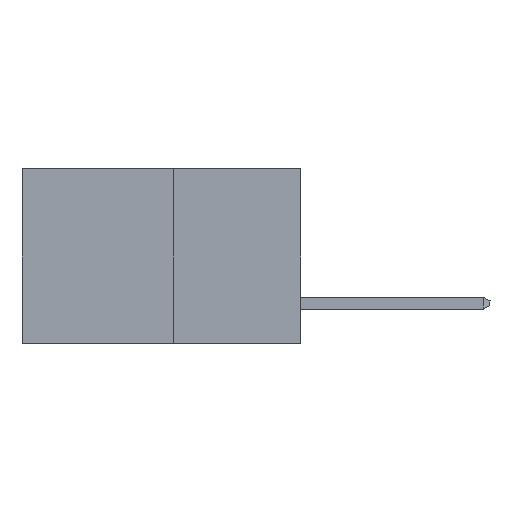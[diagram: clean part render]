
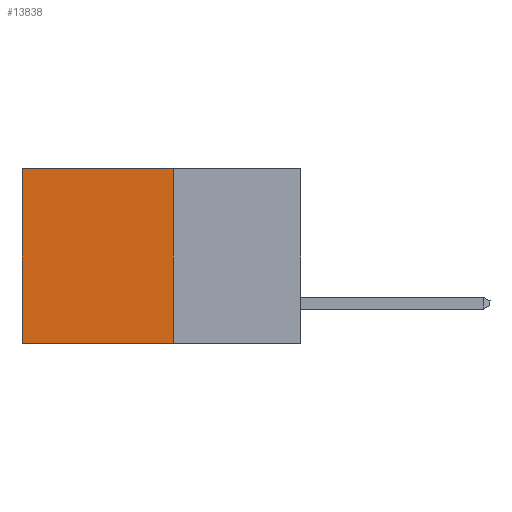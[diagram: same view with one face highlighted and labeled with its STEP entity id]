
A CAD part, left-side view. The second image highlights one B-rep face of the part: STEP entity #13838.
In plain terms, the highlighted planar face has unit normal (-1, 0, 0).
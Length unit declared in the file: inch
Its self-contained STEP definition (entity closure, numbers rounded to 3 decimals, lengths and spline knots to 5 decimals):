
#48 = CARTESIAN_POINT ( 'NONE',  ( 0.277, 0.27, -0.37 ) ) ;
#764 = EDGE_CURVE ( 'NONE', #28295, #18901, #22258, .T. ) ;
#2842 = CARTESIAN_POINT ( 'NONE',  ( 0.277, 0.59, -0.37 ) ) ;
#5871 = VERTEX_POINT ( 'NONE', #8468 ) ;
#8468 = CARTESIAN_POINT ( 'NONE',  ( 0.277, 0.27, 0. ) ) ;
#9261 = ORIENTED_EDGE ( 'NONE', *, *, #764, .F. ) ;
#9812 = DIRECTION ( 'NONE',  ( 0., 0., -1. ) ) ;
#9816 = DIRECTION ( 'NONE',  ( 1., 0., 0. ) ) ;
#9841 = PLANE ( 'NONE',  #12626 ) ;
#10137 = CARTESIAN_POINT ( 'NONE',  ( 0.277, 0.59, 0. ) ) ;
#10373 = CARTESIAN_POINT ( 'NONE',  ( 0.277, 0.27, -0.37 ) ) ;
#11152 = FACE_OUTER_BOUND ( 'NONE', #24203, .T. ) ;
#11753 = CARTESIAN_POINT ( 'NONE',  ( 0.277, 0.27, -0.37 ) ) ;
#12385 = EDGE_CURVE ( 'NONE', #5871, #28295, #22748, .T. ) ;
#12626 = AXIS2_PLACEMENT_3D ( 'NONE', #10373, #9816, #9812 ) ;
#13838 = ADVANCED_FACE ( 'NONE', ( #11152 ), #9841, .F. ) ;
#14137 = DIRECTION ( 'NONE',  ( 0., 0., -1. ) ) ;
#14610 = CARTESIAN_POINT ( 'NONE',  ( 0.277, 0.27, -0.37 ) ) ;
#16037 = VECTOR ( 'NONE', #20613, 39.37008 ) ;
#16950 = ORIENTED_EDGE ( 'NONE', *, *, #19586, .T. ) ;
#18901 = VERTEX_POINT ( 'NONE', #2842 ) ;
#19586 = EDGE_CURVE ( 'NONE', #26565, #18901, #22570, .T. ) ;
#20613 = DIRECTION ( 'NONE',  ( 0., 1., 0. ) ) ;
#20700 = EDGE_CURVE ( 'NONE', #5871, #26565, #21063, .T. ) ;
#21063 = LINE ( 'NONE', #24975, #26638 ) ;
#22012 = VECTOR ( 'NONE', #14137, 39.37008 ) ;
#22258 = LINE ( 'NONE', #11753, #16037 ) ;
#22570 = LINE ( 'NONE', #27445, #28870 ) ;
#22748 = LINE ( 'NONE', #48, #22012 ) ;
#23289 = ORIENTED_EDGE ( 'NONE', *, *, #12385, .F. ) ;
#24203 = EDGE_LOOP ( 'NONE', ( #16950, #9261, #23289, #26128 ) ) ;
#24975 = CARTESIAN_POINT ( 'NONE',  ( 0.277, 0.27, 0. ) ) ;
#25074 = DIRECTION ( 'NONE',  ( 0., 1., 0. ) ) ;
#26128 = ORIENTED_EDGE ( 'NONE', *, *, #20700, .T. ) ;
#26565 = VERTEX_POINT ( 'NONE', #10137 ) ;
#26638 = VECTOR ( 'NONE', #25074, 39.37008 ) ;
#27445 = CARTESIAN_POINT ( 'NONE',  ( 0.277, 0.59, -0.37 ) ) ;
#28295 = VERTEX_POINT ( 'NONE', #14610 ) ;
#28870 = VECTOR ( 'NONE', #29789, 39.37008 ) ;
#29789 = DIRECTION ( 'NONE',  ( 0., 0., -1. ) ) ;
